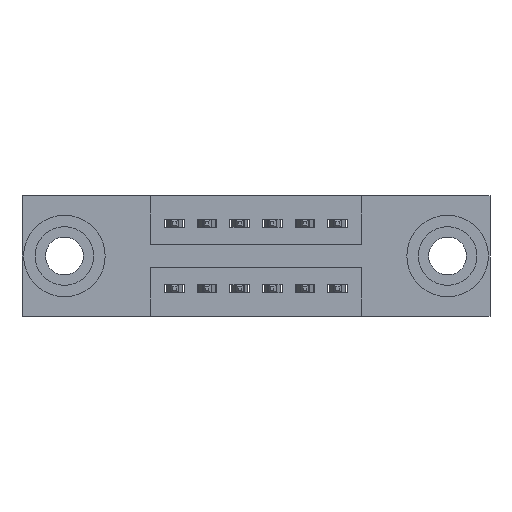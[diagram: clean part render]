
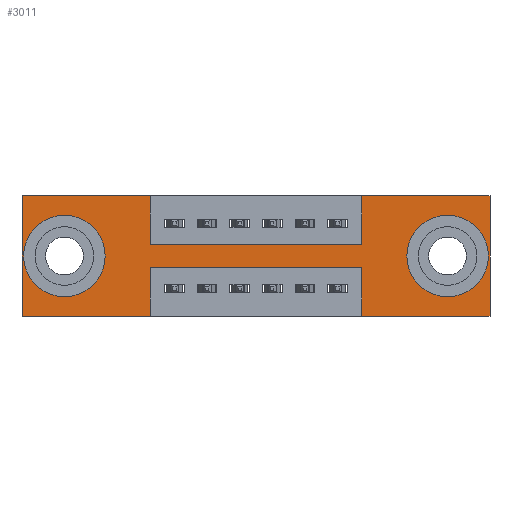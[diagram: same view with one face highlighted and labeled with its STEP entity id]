
A CAD part, front view. The second image highlights one B-rep face of the part: STEP entity #3011.
In plain terms, the highlighted planar face has unit normal (0, -1, 0).
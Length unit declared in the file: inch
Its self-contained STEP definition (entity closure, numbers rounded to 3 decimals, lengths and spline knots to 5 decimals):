
#256 = CIRCLE ( 'NONE', #9542, 0.078 ) ;
#357 = DIRECTION ( 'NONE',  ( -1., 0., 0. ) ) ;
#358 = DIRECTION ( 'NONE',  ( 0., 0., -1. ) ) ;
#443 = CARTESIAN_POINT ( 'NONE',  ( 1.435, 0., -0.37 ) ) ;
#467 = DIRECTION ( 'NONE',  ( 0., 0., -1. ) ) ;
#472 = CARTESIAN_POINT ( 'NONE',  ( 0., 0., -0.37 ) ) ;
#479 = CARTESIAN_POINT ( 'NONE',  ( 0.3925, 0., -0.37 ) ) ;
#481 = EDGE_CURVE ( 'NONE', #8792, #5239, #4222, .T. ) ;
#537 = DIRECTION ( 'NONE',  ( 0., 1., 0. ) ) ;
#568 = EDGE_CURVE ( 'NONE', #4247, #1369, #6231, .T. ) ;
#629 = VERTEX_POINT ( 'NONE', #4427 ) ;
#706 = VECTOR ( 'NONE', #4903, 39.37008 ) ;
#918 = DIRECTION ( 'NONE',  ( 0., 0., -1. ) ) ;
#979 = EDGE_CURVE ( 'NONE', #3357, #3993, #9981, .T. ) ;
#1038 = CARTESIAN_POINT ( 'NONE',  ( 0.13, 0., -0.107 ) ) ;
#1040 = LINE ( 'NONE', #4889, #9084 ) ;
#1056 = VERTEX_POINT ( 'NONE', #443 ) ;
#1194 = EDGE_CURVE ( 'NONE', #1552, #2360, #8802, .T. ) ;
#1280 = CARTESIAN_POINT ( 'NONE',  ( 0.3925, 0., -0.15 ) ) ;
#1337 = ORIENTED_EDGE ( 'NONE', *, *, #7494, .F. ) ;
#1369 = VERTEX_POINT ( 'NONE', #1038 ) ;
#1449 = CARTESIAN_POINT ( 'NONE',  ( 0.3925, 0., -0.15 ) ) ;
#1500 = ORIENTED_EDGE ( 'NONE', *, *, #8756, .T. ) ;
#1552 = VERTEX_POINT ( 'NONE', #9161 ) ;
#1564 = CARTESIAN_POINT ( 'NONE',  ( 0.3925, 0., 0. ) ) ;
#1712 = DIRECTION ( 'NONE',  ( 0., 0., -1. ) ) ;
#1728 = PLANE ( 'NONE',  #9972 ) ;
#1729 = CARTESIAN_POINT ( 'NONE',  ( 1.305, 0., -0.107 ) ) ;
#1734 = ORIENTED_EDGE ( 'NONE', *, *, #5120, .F. ) ;
#1845 = DIRECTION ( 'NONE',  ( 1., 0., 0. ) ) ;
#1876 = VERTEX_POINT ( 'NONE', #10086 ) ;
#2010 = ORIENTED_EDGE ( 'NONE', *, *, #5007, .F. ) ;
#2103 = VERTEX_POINT ( 'NONE', #8139 ) ;
#2278 = DIRECTION ( 'NONE',  ( 0., 0., 1. ) ) ;
#2360 = VERTEX_POINT ( 'NONE', #5583 ) ;
#2431 = CARTESIAN_POINT ( 'NONE',  ( 0., 0., 0. ) ) ;
#2445 = CARTESIAN_POINT ( 'NONE',  ( 1.0425, 0., -0.15 ) ) ;
#2573 = EDGE_CURVE ( 'NONE', #1876, #1552, #7950, .T. ) ;
#2594 = AXIS2_PLACEMENT_3D ( 'NONE', #7472, #3485, #5671 ) ;
#2667 = ORIENTED_EDGE ( 'NONE', *, *, #4317, .F. ) ;
#2686 = ORIENTED_EDGE ( 'NONE', *, *, #7995, .F. ) ;
#2751 = CARTESIAN_POINT ( 'NONE',  ( 1.305, 0., -0.185 ) ) ;
#2762 = DIRECTION ( 'NONE',  ( 1., 0., 0. ) ) ;
#2827 = EDGE_CURVE ( 'NONE', #2103, #9070, #3934, .T. ) ;
#3011 = ADVANCED_FACE ( 'NONE', ( #4312, #4554, #10210 ), #1728, .T. ) ;
#3043 = ORIENTED_EDGE ( 'NONE', *, *, #6432, .F. ) ;
#3127 = LINE ( 'NONE', #1564, #4987 ) ;
#3280 = ORIENTED_EDGE ( 'NONE', *, *, #979, .F. ) ;
#3357 = VERTEX_POINT ( 'NONE', #1280 ) ;
#3485 = DIRECTION ( 'NONE',  ( 0., 1., 0. ) ) ;
#3644 = ORIENTED_EDGE ( 'NONE', *, *, #5961, .T. ) ;
#3745 = ORIENTED_EDGE ( 'NONE', *, *, #481, .T. ) ;
#3934 = LINE ( 'NONE', #479, #9605 ) ;
#3955 = LINE ( 'NONE', #8305, #5675 ) ;
#3993 = VERTEX_POINT ( 'NONE', #2445 ) ;
#4038 = VECTOR ( 'NONE', #8236, 39.37008 ) ;
#4222 = CIRCLE ( 'NONE', #4422, 0.078 ) ;
#4247 = VERTEX_POINT ( 'NONE', #8558 ) ;
#4312 = FACE_BOUND ( 'NONE', #6087, .T. ) ;
#4317 = EDGE_CURVE ( 'NONE', #9089, #9633, #9695, .T. ) ;
#4422 = AXIS2_PLACEMENT_3D ( 'NONE', #2751, #8047, #8977 ) ;
#4427 = CARTESIAN_POINT ( 'NONE',  ( 1.435, 0., 0. ) ) ;
#4461 = ORIENTED_EDGE ( 'NONE', *, *, #8588, .F. ) ;
#4471 = ORIENTED_EDGE ( 'NONE', *, *, #2827, .F. ) ;
#4554 = FACE_BOUND ( 'NONE', #6204, .T. ) ;
#4570 = ORIENTED_EDGE ( 'NONE', *, *, #568, .T. ) ;
#4803 = DIRECTION ( 'NONE',  ( 0., 0., 1. ) ) ;
#4889 = CARTESIAN_POINT ( 'NONE',  ( 1.0425, 0., 0. ) ) ;
#4903 = DIRECTION ( 'NONE',  ( -1., 0., 0. ) ) ;
#4962 = CIRCLE ( 'NONE', #8661, 0.078 ) ;
#4987 = VECTOR ( 'NONE', #1712, 39.37008 ) ;
#5007 = EDGE_CURVE ( 'NONE', #2360, #3357, #3127, .T. ) ;
#5029 = CARTESIAN_POINT ( 'NONE',  ( 0.3925, 0., -0.37 ) ) ;
#5091 = ORIENTED_EDGE ( 'NONE', *, *, #5314, .F. ) ;
#5120 = EDGE_CURVE ( 'NONE', #9070, #1876, #5742, .T. ) ;
#5164 = DIRECTION ( 'NONE',  ( 0., 0., 1. ) ) ;
#5239 = VERTEX_POINT ( 'NONE', #1729 ) ;
#5240 = CARTESIAN_POINT ( 'NONE',  ( 0., 0., 0. ) ) ;
#5307 = VERTEX_POINT ( 'NONE', #7749 ) ;
#5314 = EDGE_CURVE ( 'NONE', #1056, #9089, #10058, .T. ) ;
#5317 = ORIENTED_EDGE ( 'NONE', *, *, #2573, .F. ) ;
#5374 = ORIENTED_EDGE ( 'NONE', *, *, #1194, .F. ) ;
#5493 = CARTESIAN_POINT ( 'NONE',  ( 1.305, 0., -0.185 ) ) ;
#5583 = CARTESIAN_POINT ( 'NONE',  ( 0.3925, 0., 0. ) ) ;
#5606 = CARTESIAN_POINT ( 'NONE',  ( 0.3925, 0., -0.22 ) ) ;
#5671 = DIRECTION ( 'NONE',  ( 0., 0., 1. ) ) ;
#5675 = VECTOR ( 'NONE', #358, 39.37008 ) ;
#5742 = LINE ( 'NONE', #472, #9468 ) ;
#5931 = EDGE_LOOP ( 'NONE', ( #4471, #1337, #2667, #5091, #4461, #2686, #3043, #3280, #2010, #5374, #5317, #1734 ) ) ;
#5961 = EDGE_CURVE ( 'NONE', #1369, #4247, #4962, .T. ) ;
#6087 = EDGE_LOOP ( 'NONE', ( #1500, #3745 ) ) ;
#6204 = EDGE_LOOP ( 'NONE', ( #3644, #4570 ) ) ;
#6206 = DIRECTION ( 'NONE',  ( 0., 0., -1. ) ) ;
#6231 = CIRCLE ( 'NONE', #2594, 0.078 ) ;
#6432 = EDGE_CURVE ( 'NONE', #3993, #5307, #1040, .T. ) ;
#6525 = CARTESIAN_POINT ( 'NONE',  ( 1.0425, 0., -0.37 ) ) ;
#6827 = VECTOR ( 'NONE', #9130, 39.37008 ) ;
#6874 = CARTESIAN_POINT ( 'NONE',  ( 0., 0., 0. ) ) ;
#7078 = LINE ( 'NONE', #5606, #706 ) ;
#7297 = LINE ( 'NONE', #6874, #6827 ) ;
#7356 = DIRECTION ( 'NONE',  ( -1., 0., 0. ) ) ;
#7472 = CARTESIAN_POINT ( 'NONE',  ( 0.13, 0., -0.185 ) ) ;
#7494 = EDGE_CURVE ( 'NONE', #9633, #2103, #7078, .T. ) ;
#7621 = VECTOR ( 'NONE', #2762, 39.37008 ) ;
#7749 = CARTESIAN_POINT ( 'NONE',  ( 1.0425, 0., 0. ) ) ;
#7816 = CARTESIAN_POINT ( 'NONE',  ( 0., 0., -0.37 ) ) ;
#7950 = LINE ( 'NONE', #2431, #9955 ) ;
#7980 = CARTESIAN_POINT ( 'NONE',  ( 1.0425, 0., -0.22 ) ) ;
#7995 = EDGE_CURVE ( 'NONE', #5307, #629, #7297, .T. ) ;
#8005 = DIRECTION ( 'NONE',  ( 0., -1., 0. ) ) ;
#8037 = VECTOR ( 'NONE', #7356, 39.37008 ) ;
#8047 = DIRECTION ( 'NONE',  ( 0., 1., 0. ) ) ;
#8139 = CARTESIAN_POINT ( 'NONE',  ( 0.3925, 0., -0.22 ) ) ;
#8236 = DIRECTION ( 'NONE',  ( 0., 0., 1. ) ) ;
#8267 = CARTESIAN_POINT ( 'NONE',  ( 1.0425, 0., -0.37 ) ) ;
#8305 = CARTESIAN_POINT ( 'NONE',  ( 1.435, 0., 0. ) ) ;
#8558 = CARTESIAN_POINT ( 'NONE',  ( 0.13, 0., -0.263 ) ) ;
#8588 = EDGE_CURVE ( 'NONE', #629, #1056, #3955, .T. ) ;
#8661 = AXIS2_PLACEMENT_3D ( 'NONE', #9987, #9583, #5164 ) ;
#8756 = EDGE_CURVE ( 'NONE', #5239, #8792, #256, .T. ) ;
#8792 = VERTEX_POINT ( 'NONE', #9212 ) ;
#8802 = LINE ( 'NONE', #5240, #7621 ) ;
#8803 = CARTESIAN_POINT ( 'NONE',  ( 0., 0., -0.37 ) ) ;
#8977 = DIRECTION ( 'NONE',  ( 0., 0., -1. ) ) ;
#9035 = VECTOR ( 'NONE', #1845, 39.37008 ) ;
#9070 = VERTEX_POINT ( 'NONE', #5029 ) ;
#9084 = VECTOR ( 'NONE', #4803, 39.37008 ) ;
#9089 = VERTEX_POINT ( 'NONE', #6525 ) ;
#9130 = DIRECTION ( 'NONE',  ( 1., 0., 0. ) ) ;
#9161 = CARTESIAN_POINT ( 'NONE',  ( 0., 0., 0. ) ) ;
#9212 = CARTESIAN_POINT ( 'NONE',  ( 1.305, 0., -0.263 ) ) ;
#9468 = VECTOR ( 'NONE', #357, 39.37008 ) ;
#9542 = AXIS2_PLACEMENT_3D ( 'NONE', #5493, #537, #6206 ) ;
#9583 = DIRECTION ( 'NONE',  ( 0., 1., 0. ) ) ;
#9605 = VECTOR ( 'NONE', #467, 39.37008 ) ;
#9633 = VERTEX_POINT ( 'NONE', #7980 ) ;
#9695 = LINE ( 'NONE', #8267, #4038 ) ;
#9955 = VECTOR ( 'NONE', #2278, 39.37008 ) ;
#9972 = AXIS2_PLACEMENT_3D ( 'NONE', #8803, #8005, #918 ) ;
#9981 = LINE ( 'NONE', #1449, #9035 ) ;
#9987 = CARTESIAN_POINT ( 'NONE',  ( 0.13, 0., -0.185 ) ) ;
#10058 = LINE ( 'NONE', #7816, #8037 ) ;
#10086 = CARTESIAN_POINT ( 'NONE',  ( 0., 0., -0.37 ) ) ;
#10210 = FACE_OUTER_BOUND ( 'NONE', #5931, .T. ) ;
